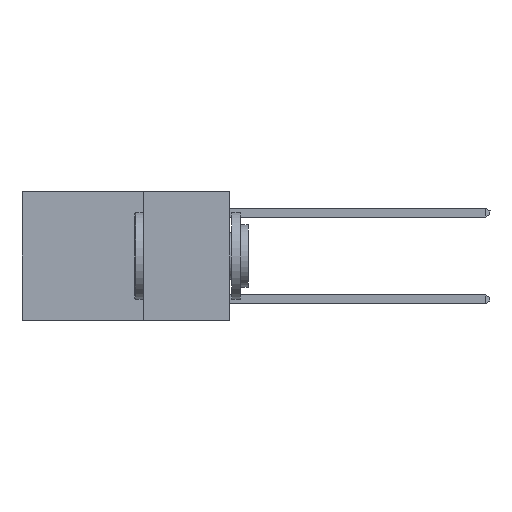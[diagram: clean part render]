
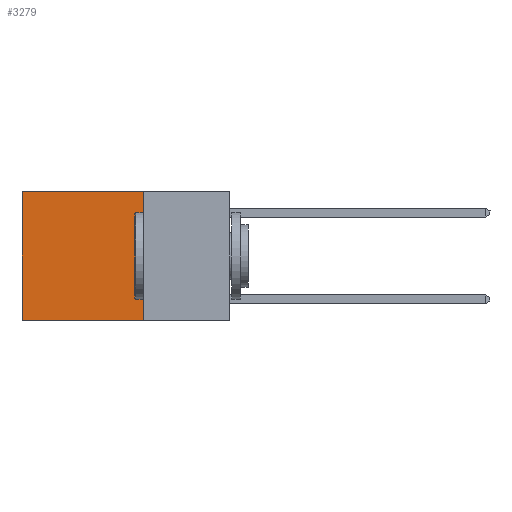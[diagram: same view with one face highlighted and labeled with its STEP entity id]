
A CAD part, left-side view. The second image highlights one B-rep face of the part: STEP entity #3279.
In plain terms, the highlighted planar face has unit normal (-1, 0, 0).
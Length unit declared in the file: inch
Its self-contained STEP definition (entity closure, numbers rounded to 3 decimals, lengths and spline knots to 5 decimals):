
#61 = VERTEX_POINT ( 'NONE', #7028 ) ;
#437 = DIRECTION ( 'NONE',  ( 0., 1., 0. ) ) ;
#546 = LINE ( 'NONE', #19101, #2673 ) ;
#1073 = VECTOR ( 'NONE', #3945, 39.37008 ) ;
#1297 = EDGE_CURVE ( 'NONE', #15560, #21728, #17742, .T. ) ;
#1383 = VERTEX_POINT ( 'NONE', #16847 ) ;
#2429 = DIRECTION ( 'NONE',  ( 0., 1., 0. ) ) ;
#2673 = VECTOR ( 'NONE', #437, 39.37008 ) ;
#2730 = DIRECTION ( 'NONE',  ( 0., 0., -1. ) ) ;
#3279 = ADVANCED_FACE ( 'NONE', ( #21866 ), #20077, .F. ) ;
#3463 = EDGE_LOOP ( 'NONE', ( #12513, #12615, #17468, #16362 ) ) ;
#3945 = DIRECTION ( 'NONE',  ( 0., 0., -1. ) ) ;
#4232 = LINE ( 'NONE', #11062, #15549 ) ;
#5003 = EDGE_CURVE ( 'NONE', #21728, #1383, #4232, .T. ) ;
#5153 = VECTOR ( 'NONE', #2730, 39.37008 ) ;
#7028 = CARTESIAN_POINT ( 'NONE',  ( 0.2625, 0.6, 0. ) ) ;
#7182 = CARTESIAN_POINT ( 'NONE',  ( 0.2625, 0.25, -0.37 ) ) ;
#7849 = LINE ( 'NONE', #14840, #5153 ) ;
#8474 = CARTESIAN_POINT ( 'NONE',  ( 0.2625, 0.25, 0. ) ) ;
#9930 = EDGE_CURVE ( 'NONE', #61, #1383, #7849, .T. ) ;
#11062 = CARTESIAN_POINT ( 'NONE',  ( 0.2625, 0.25, -0.37 ) ) ;
#11641 = DIRECTION ( 'NONE',  ( 1., 0., 0. ) ) ;
#11841 = AXIS2_PLACEMENT_3D ( 'NONE', #8474, #11641, #16822 ) ;
#12513 = ORIENTED_EDGE ( 'NONE', *, *, #9930, .T. ) ;
#12615 = ORIENTED_EDGE ( 'NONE', *, *, #5003, .F. ) ;
#13455 = EDGE_CURVE ( 'NONE', #15560, #61, #546, .T. ) ;
#14840 = CARTESIAN_POINT ( 'NONE',  ( 0.2625, 0.6, 0. ) ) ;
#15549 = VECTOR ( 'NONE', #2429, 39.37008 ) ;
#15560 = VERTEX_POINT ( 'NONE', #18681 ) ;
#16362 = ORIENTED_EDGE ( 'NONE', *, *, #13455, .T. ) ;
#16822 = DIRECTION ( 'NONE',  ( 0., 0., -1. ) ) ;
#16847 = CARTESIAN_POINT ( 'NONE',  ( 0.2625, 0.6, -0.37 ) ) ;
#17468 = ORIENTED_EDGE ( 'NONE', *, *, #1297, .F. ) ;
#17742 = LINE ( 'NONE', #21662, #1073 ) ;
#18681 = CARTESIAN_POINT ( 'NONE',  ( 0.2625, 0.25, 0. ) ) ;
#19101 = CARTESIAN_POINT ( 'NONE',  ( 0.2625, 0.25, 0. ) ) ;
#20077 = PLANE ( 'NONE',  #11841 ) ;
#21662 = CARTESIAN_POINT ( 'NONE',  ( 0.2625, 0.25, 0. ) ) ;
#21728 = VERTEX_POINT ( 'NONE', #7182 ) ;
#21866 = FACE_OUTER_BOUND ( 'NONE', #3463, .T. ) ;
